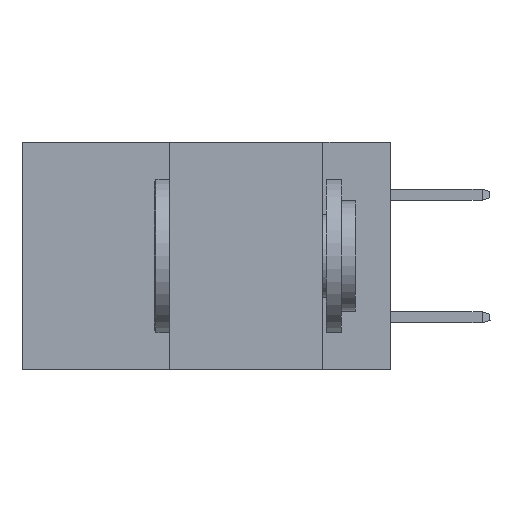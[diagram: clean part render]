
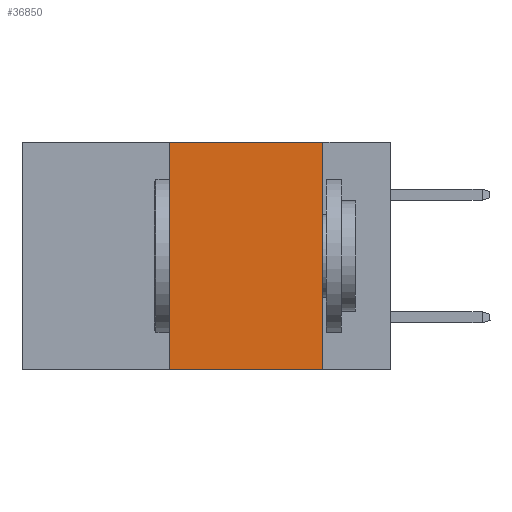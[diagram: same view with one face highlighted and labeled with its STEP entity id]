
A CAD part, left-side view. The second image highlights one B-rep face of the part: STEP entity #36850.
In plain terms, the highlighted planar face has unit normal (-1, 0, 0).
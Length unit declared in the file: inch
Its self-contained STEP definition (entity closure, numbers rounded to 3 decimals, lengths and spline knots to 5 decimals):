
#911 = ORIENTED_EDGE ( 'NONE', *, *, #18826, .F. ) ;
#1922 = ORIENTED_EDGE ( 'NONE', *, *, #18285, .F. ) ;
#2161 = CARTESIAN_POINT ( 'NONE',  ( 0., 0.36, -0.37 ) ) ;
#4391 = CARTESIAN_POINT ( 'NONE',  ( 0., 0.11, 0. ) ) ;
#5567 = VERTEX_POINT ( 'NONE', #13596 ) ;
#5887 = CARTESIAN_POINT ( 'NONE',  ( 0., 0.11, 0. ) ) ;
#7207 = CARTESIAN_POINT ( 'NONE',  ( 0., 0.36, 0. ) ) ;
#9330 = ORIENTED_EDGE ( 'NONE', *, *, #14123, .T. ) ;
#10299 = LINE ( 'NONE', #4391, #29532 ) ;
#10919 = VERTEX_POINT ( 'NONE', #31876 ) ;
#11173 = CARTESIAN_POINT ( 'NONE',  ( 0., 0.6, -0.37 ) ) ;
#11357 = LINE ( 'NONE', #11173, #12876 ) ;
#12876 = VECTOR ( 'NONE', #21224, 39.37008 ) ;
#13596 = CARTESIAN_POINT ( 'NONE',  ( 0., 0.36, 0. ) ) ;
#13668 = DIRECTION ( 'NONE',  ( 0., -1., 0. ) ) ;
#14123 = EDGE_CURVE ( 'NONE', #38300, #10919, #11357, .T. ) ;
#16283 = VERTEX_POINT ( 'NONE', #5887 ) ;
#17334 = AXIS2_PLACEMENT_3D ( 'NONE', #37666, #21157, #20869 ) ;
#17728 = DIRECTION ( 'NONE',  ( 0., 0., -1. ) ) ;
#18017 = VECTOR ( 'NONE', #13668, 39.37008 ) ;
#18285 = EDGE_CURVE ( 'NONE', #38300, #5567, #25845, .T. ) ;
#18826 = EDGE_CURVE ( 'NONE', #5567, #16283, #29975, .T. ) ;
#20869 = DIRECTION ( 'NONE',  ( 0., 0., -1. ) ) ;
#21010 = PLANE ( 'NONE',  #17334 ) ;
#21157 = DIRECTION ( 'NONE',  ( 1., 0., 0. ) ) ;
#21224 = DIRECTION ( 'NONE',  ( 0., -1., 0. ) ) ;
#25845 = LINE ( 'NONE', #7207, #34670 ) ;
#29532 = VECTOR ( 'NONE', #17728, 39.37008 ) ;
#29975 = LINE ( 'NONE', #39973, #18017 ) ;
#31876 = CARTESIAN_POINT ( 'NONE',  ( 0., 0.11, -0.37 ) ) ;
#33158 = EDGE_CURVE ( 'NONE', #16283, #10919, #10299, .T. ) ;
#34036 = ORIENTED_EDGE ( 'NONE', *, *, #33158, .F. ) ;
#34181 = DIRECTION ( 'NONE',  ( 0., 0., 1. ) ) ;
#34670 = VECTOR ( 'NONE', #34181, 39.37008 ) ;
#36188 = FACE_OUTER_BOUND ( 'NONE', #40059, .T. ) ;
#36850 = ADVANCED_FACE ( 'NONE', ( #36188 ), #21010, .F. ) ;
#37666 = CARTESIAN_POINT ( 'NONE',  ( 0., 0.6, 0. ) ) ;
#38300 = VERTEX_POINT ( 'NONE', #2161 ) ;
#39973 = CARTESIAN_POINT ( 'NONE',  ( 0., 0.6, 0. ) ) ;
#40059 = EDGE_LOOP ( 'NONE', ( #34036, #911, #1922, #9330 ) ) ;
